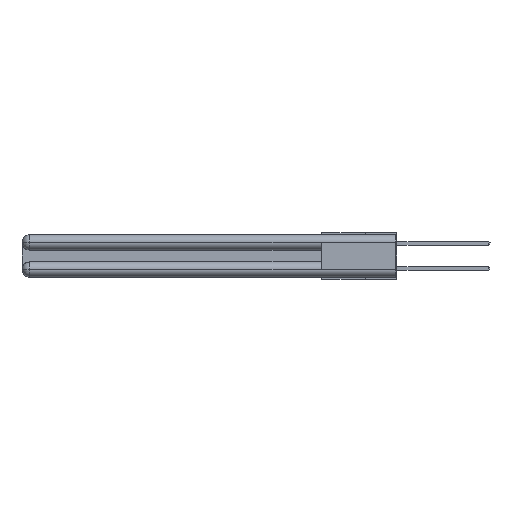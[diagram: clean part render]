
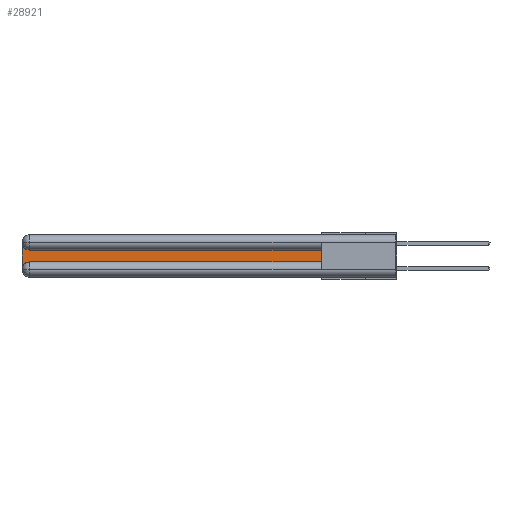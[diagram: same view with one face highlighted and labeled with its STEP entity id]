
A CAD part, left-side view. The second image highlights one B-rep face of the part: STEP entity #28921.
In plain terms, the highlighted planar face has unit normal (-1, 0, 0).
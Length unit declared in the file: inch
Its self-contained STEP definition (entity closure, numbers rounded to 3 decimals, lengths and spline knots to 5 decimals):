
#910 = EDGE_CURVE ( 'NONE', #14453, #20966, #11425, .T. ) ;
#3295 = LINE ( 'NONE', #18378, #31992 ) ;
#3323 = DIRECTION ( 'NONE',  ( 0., 0., -1. ) ) ;
#3610 = DIRECTION ( 'NONE',  ( 0., 0., -1. ) ) ;
#4435 = ORIENTED_EDGE ( 'NONE', *, *, #29496, .T. ) ;
#4931 = VERTEX_POINT ( 'NONE', #5262 ) ;
#5262 = CARTESIAN_POINT ( 'NONE',  ( 0.075, 2.94, -0.2175 ) ) ;
#5410 = EDGE_LOOP ( 'NONE', ( #24810, #22885, #29216, #4435, #31166, #25230 ) ) ;
#6713 = DIRECTION ( 'NONE',  ( 0., 1., 0. ) ) ;
#6776 = CARTESIAN_POINT ( 'NONE',  ( 0.075, 3., -0.0625 ) ) ;
#7825 = DIRECTION ( 'NONE',  ( 0., 0., 1. ) ) ;
#7967 = VERTEX_POINT ( 'NONE', #8846 ) ;
#8159 = CARTESIAN_POINT ( 'NONE',  ( 0.075, 0.6, -0.2175 ) ) ;
#8553 = CARTESIAN_POINT ( 'NONE',  ( 0.075, 3., -0.2175 ) ) ;
#8846 = CARTESIAN_POINT ( 'NONE',  ( 0.075, 0.6, -0.1225 ) ) ;
#10753 = PLANE ( 'NONE',  #18037 ) ;
#11293 = CARTESIAN_POINT ( 'NONE',  ( 0.075, 2.94, -0.2775 ) ) ;
#11425 = CIRCLE ( 'NONE', #17329, 0.06 ) ;
#11542 = DIRECTION ( 'NONE',  ( 0., 0., -1. ) ) ;
#12151 = CIRCLE ( 'NONE', #29917, 0.06 ) ;
#12339 = CARTESIAN_POINT ( 'NONE',  ( 0.075, 0.6, -0.1225 ) ) ;
#12814 = VECTOR ( 'NONE', #24006, 39.37008 ) ;
#13535 = EDGE_CURVE ( 'NONE', #7967, #14453, #14723, .T. ) ;
#14041 = DIRECTION ( 'NONE',  ( 1., 0., 0. ) ) ;
#14453 = VERTEX_POINT ( 'NONE', #17513 ) ;
#14723 = LINE ( 'NONE', #12339, #27866 ) ;
#15285 = EDGE_CURVE ( 'NONE', #20966, #26425, #28970, .T. ) ;
#16350 = CARTESIAN_POINT ( 'NONE',  ( 0.075, 0.6, -0.2175 ) ) ;
#17329 = AXIS2_PLACEMENT_3D ( 'NONE', #19681, #14041, #3610 ) ;
#17513 = CARTESIAN_POINT ( 'NONE',  ( 0.075, 2.94, -0.1225 ) ) ;
#17893 = VECTOR ( 'NONE', #11542, 39.37008 ) ;
#18037 = AXIS2_PLACEMENT_3D ( 'NONE', #25986, #29062, #31452 ) ;
#18378 = CARTESIAN_POINT ( 'NONE',  ( 0.075, 0.6, -0.2175 ) ) ;
#19681 = CARTESIAN_POINT ( 'NONE',  ( 0.075, 2.94, -0.0625 ) ) ;
#20966 = VERTEX_POINT ( 'NONE', #6776 ) ;
#22885 = ORIENTED_EDGE ( 'NONE', *, *, #910, .T. ) ;
#24006 = DIRECTION ( 'NONE',  ( 0., -1., 0. ) ) ;
#24810 = ORIENTED_EDGE ( 'NONE', *, *, #13535, .T. ) ;
#25230 = ORIENTED_EDGE ( 'NONE', *, *, #25852, .T. ) ;
#25256 = FACE_OUTER_BOUND ( 'NONE', #5410, .T. ) ;
#25446 = EDGE_CURVE ( 'NONE', #4931, #26973, #26750, .T. ) ;
#25852 = EDGE_CURVE ( 'NONE', #26973, #7967, #3295, .T. ) ;
#25986 = CARTESIAN_POINT ( 'NONE',  ( 0.075, 3., -0.1225 ) ) ;
#26090 = CARTESIAN_POINT ( 'NONE',  ( 0.075, 3., -0.2775 ) ) ;
#26425 = VERTEX_POINT ( 'NONE', #26090 ) ;
#26750 = LINE ( 'NONE', #16350, #12814 ) ;
#26973 = VERTEX_POINT ( 'NONE', #8159 ) ;
#27866 = VECTOR ( 'NONE', #6713, 39.37008 ) ;
#28921 = ADVANCED_FACE ( 'NONE', ( #25256 ), #10753, .F. ) ;
#28970 = LINE ( 'NONE', #8553, #17893 ) ;
#29062 = DIRECTION ( 'NONE',  ( 1., 0., 0. ) ) ;
#29216 = ORIENTED_EDGE ( 'NONE', *, *, #15285, .T. ) ;
#29496 = EDGE_CURVE ( 'NONE', #26425, #4931, #12151, .T. ) ;
#29917 = AXIS2_PLACEMENT_3D ( 'NONE', #11293, #32074, #3323 ) ;
#31166 = ORIENTED_EDGE ( 'NONE', *, *, #25446, .T. ) ;
#31452 = DIRECTION ( 'NONE',  ( 0., 0., -1. ) ) ;
#31992 = VECTOR ( 'NONE', #7825, 39.37008 ) ;
#32074 = DIRECTION ( 'NONE',  ( 1., 0., 0. ) ) ;
